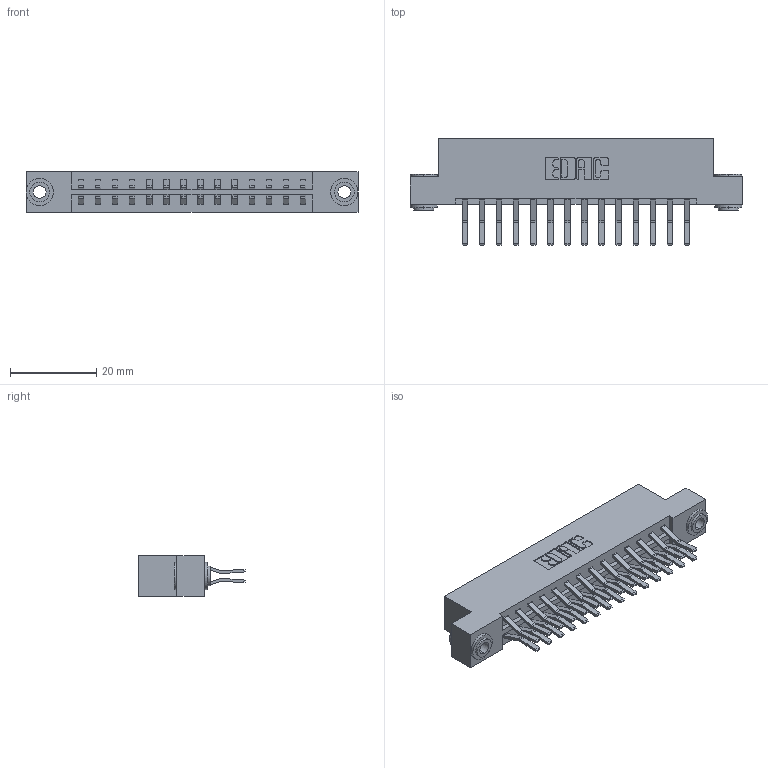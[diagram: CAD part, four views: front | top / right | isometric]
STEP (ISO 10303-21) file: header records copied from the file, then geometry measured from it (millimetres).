
FILE_DESCRIPTION (( 'STEP AP203' ), '1' );
FILE_NAME ('333-028-560-203.STEP', '2018-08-02T16:01:54', ( '' ), ( '' ), 'SwSTEP 2.0', 'SolidWorks 2016', '' );
FILE_SCHEMA (( 'CONFIG_CONTROL_DESIGN' ));
Length unit declared in the file: inch
Products named in the file (4): 333 Part_Flush - .156 Dia - TH; 345-292-001_560 Tail; 345-250-002_345-250-002-102; 333-028-560-203
Assembly tree (31 placements, depth 2):
  333-028-560-203
    333 Part_Flush - .156 Dia - TH
    345-292-001_560 Tail  x28
    345-250-002_345-250-002-102  x2
Bounding box: 77.01 x 24.78 x 9.4 mm (x, y, z)
Volume: 7803.6 mm3; surface area: 9669.4 mm2
Topology: 31 solids, 31 shells, 1664 faces, 4895 edges, 3222 vertices
Faces by surface type: plane 1088, cylinder 568, cone 8
Entity records: 13366 total; most frequent: CARTESIAN_POINT 2225, ORIENTED_EDGE 2154, DIRECTION 1987, EDGE_CURVE 1077, LINE 921, VECTOR 921, VERTEX_POINT 714, AXIS2_PLACEMENT_3D 533
